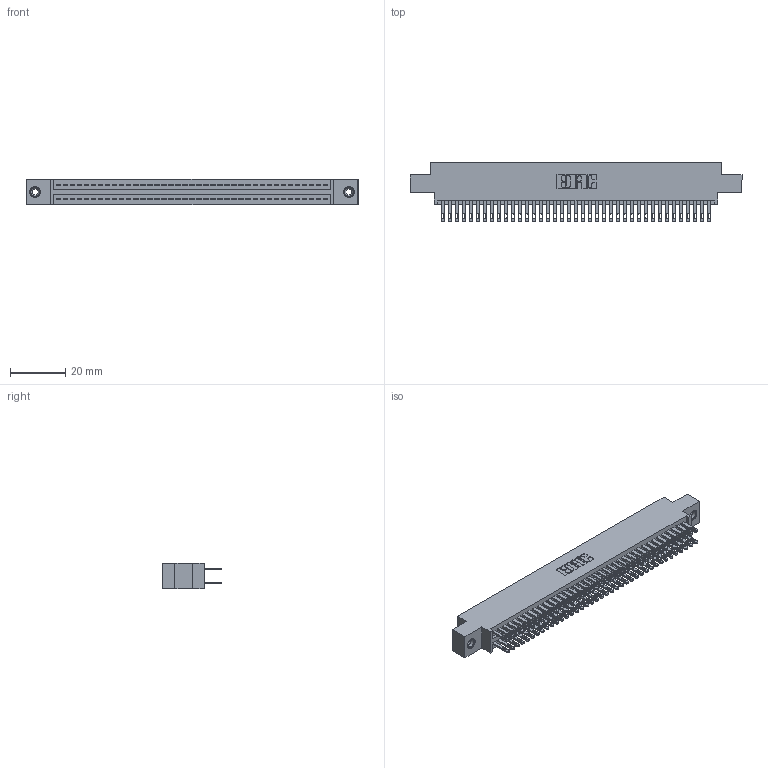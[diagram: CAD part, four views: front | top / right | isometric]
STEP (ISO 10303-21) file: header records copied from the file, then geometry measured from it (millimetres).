
FILE_DESCRIPTION (( 'STEP AP203' ), '1' );
FILE_NAME ('345-078-500-808.STEP', '2019-10-31T14:32:31', ( '' ), ( '' ), 'SwSTEP 2.0', 'SolidWorks 2016', '' );
FILE_SCHEMA (( 'CONFIG_CONTROL_DESIGN' ));
Length unit declared in the file: inch
Products named in the file (4): 345-078-500-808; 345 Part_0.170 Offset - 0.156 Dia-TI; 345-292-001_345-293-100; 345-250-001_345-250-003-102
Assembly tree (81 placements, depth 2):
  345-078-500-808
    345 Part_0.170 Offset - 0.156 Dia-TI
    345-292-001_345-293-100  x78
    345-250-001_345-250-003-102  x2
Bounding box: 120.27 x 21.51 x 9.4 mm (x, y, z)
Volume: 11773.7 mm3; surface area: 18297.8 mm2
Topology: 81 solids, 81 shells, 3778 faces, 11487 edges, 7650 vertices
Faces by surface type: plane 2222, cylinder 1540, cone 12, torus 4
Entity records: 32252 total; most frequent: CARTESIAN_POINT 5391, ORIENTED_EDGE 5318, DIRECTION 4785, EDGE_CURVE 2659, LINE 2347, VECTOR 2347, VERTEX_POINT 1768, AXIS2_PLACEMENT_3D 1219
